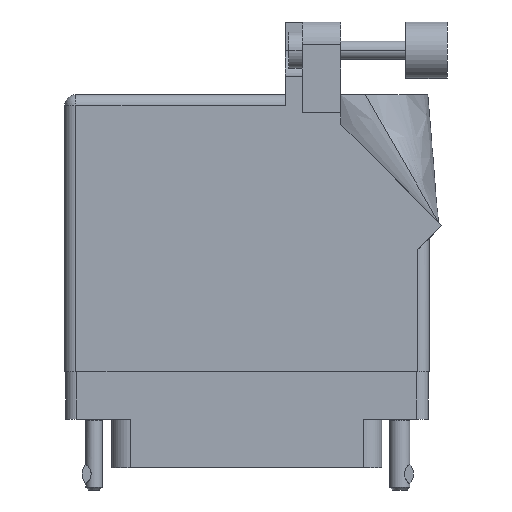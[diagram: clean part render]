
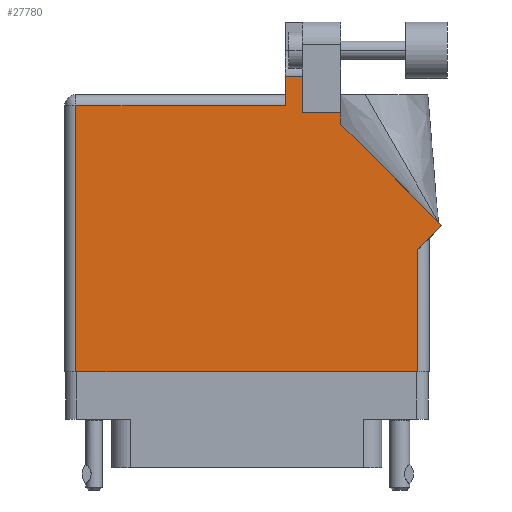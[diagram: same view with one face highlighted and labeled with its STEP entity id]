
A CAD part, front view. The second image highlights one B-rep face of the part: STEP entity #27780.
In plain terms, the highlighted face is planar.
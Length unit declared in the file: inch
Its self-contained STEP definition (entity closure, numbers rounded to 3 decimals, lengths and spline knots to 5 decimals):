
#289 = VECTOR ( 'NONE', #42647, 39.37008 ) ;
#941 = DIRECTION ( 'NONE',  ( 0.707, 0.707, 0. ) ) ;
#992 = DIRECTION ( 'NONE',  ( -0.707, 0.707, 0. ) ) ;
#1466 = VERTEX_POINT ( 'NONE', #11224 ) ;
#1578 = VERTEX_POINT ( 'NONE', #34021 ) ;
#2413 = CARTESIAN_POINT ( 'NONE',  ( 0.062, 0., 0. ) ) ;
#2607 = CARTESIAN_POINT ( 'NONE',  ( 0., 1.53, 0. ) ) ;
#2771 = CARTESIAN_POINT ( 'NONE',  ( 1.64177, 1.6315, 0. ) ) ;
#3176 = LINE ( 'NONE', #9819, #13728 ) ;
#3373 = CARTESIAN_POINT ( 'NONE',  ( 0.062, 0., 0. ) ) ;
#3840 = VECTOR ( 'NONE', #33177, 39.37008 ) ;
#4231 = CARTESIAN_POINT ( 'NONE',  ( 2.01, 0.737, 0. ) ) ;
#5303 = ORIENTED_EDGE ( 'NONE', *, *, #8997, .T. ) ;
#5858 = ORIENTED_EDGE ( 'NONE', *, *, #14724, .T. ) ;
#6082 = EDGE_CURVE ( 'NONE', #47226, #1578, #3176, .T. ) ;
#6361 = LINE ( 'NONE', #26943, #45151 ) ;
#6566 = VERTEX_POINT ( 'NONE', #8274 ) ;
#6800 = CARTESIAN_POINT ( 'NONE',  ( 1.948, 0., 0. ) ) ;
#7767 = VECTOR ( 'NONE', #44574, 39.37008 ) ;
#7984 = LINE ( 'NONE', #3373, #37357 ) ;
#8274 = CARTESIAN_POINT ( 'NONE',  ( 1.217, 1.6315, 0. ) ) ;
#8997 = EDGE_CURVE ( 'NONE', #36861, #6566, #24443, .T. ) ;
#9522 = CARTESIAN_POINT ( 'NONE',  ( 1.948, 0.737, 0. ) ) ;
#9819 = CARTESIAN_POINT ( 'NONE',  ( 1.524, 1.43, 0. ) ) ;
#11224 = CARTESIAN_POINT ( 'NONE',  ( 2.08071, 0.80771, 0. ) ) ;
#11694 = LINE ( 'NONE', #4231, #39904 ) ;
#11801 = CARTESIAN_POINT ( 'NONE',  ( 0.062, 1.468, 0. ) ) ;
#11880 = AXIS2_PLACEMENT_3D ( 'NONE', #2607, #36283, #40048 ) ;
#12091 = ORIENTED_EDGE ( 'NONE', *, *, #28005, .T. ) ;
#12323 = LINE ( 'NONE', #9522, #28180 ) ;
#13728 = VECTOR ( 'NONE', #17634, 39.37008 ) ;
#14170 = VECTOR ( 'NONE', #42451, 39.37008 ) ;
#14499 = CARTESIAN_POINT ( 'NONE',  ( 1.217, 1.468, 0. ) ) ;
#14584 = VECTOR ( 'NONE', #992, 39.37008 ) ;
#14724 = EDGE_CURVE ( 'NONE', #21528, #36771, #12323, .T. ) ;
#16318 = EDGE_CURVE ( 'NONE', #6566, #29069, #6361, .T. ) ;
#17285 = ORIENTED_EDGE ( 'NONE', *, *, #37833, .T. ) ;
#17634 = DIRECTION ( 'NONE',  ( -1., 0., 0. ) ) ;
#17967 = DIRECTION ( 'NONE',  ( 0., -1., 0. ) ) ;
#19061 = EDGE_CURVE ( 'NONE', #47402, #23851, #7984, .T. ) ;
#19409 = EDGE_CURVE ( 'NONE', #43806, #47226, #36724, .T. ) ;
#21252 = LINE ( 'NONE', #36709, #7767 ) ;
#21528 = VERTEX_POINT ( 'NONE', #6800 ) ;
#21964 = CARTESIAN_POINT ( 'NONE',  ( 1.524, 1.43, 0. ) ) ;
#22410 = EDGE_CURVE ( 'NONE', #23851, #21528, #24126, .T. ) ;
#23104 = DIRECTION ( 'NONE',  ( 0., -1., 0. ) ) ;
#23851 = VERTEX_POINT ( 'NONE', #2413 ) ;
#24126 = LINE ( 'NONE', #31111, #14170 ) ;
#24443 = LINE ( 'NONE', #2771, #34416 ) ;
#24554 = LINE ( 'NONE', #41409, #14584 ) ;
#24637 = EDGE_CURVE ( 'NONE', #29069, #47402, #41446, .T. ) ;
#25114 = PLANE ( 'NONE',  #11880 ) ;
#26943 = CARTESIAN_POINT ( 'NONE',  ( 1.217, 1.53, 0. ) ) ;
#27780 = ADVANCED_FACE ( 'NONE', ( #30115 ), #25114, .F. ) ;
#28005 = EDGE_CURVE ( 'NONE', #1578, #36861, #21252, .T. ) ;
#28180 = VECTOR ( 'NONE', #35762, 39.37008 ) ;
#29069 = VERTEX_POINT ( 'NONE', #14499 ) ;
#30115 = FACE_OUTER_BOUND ( 'NONE', #38236, .T. ) ;
#31111 = CARTESIAN_POINT ( 'NONE',  ( 0., 0., 0. ) ) ;
#32686 = ORIENTED_EDGE ( 'NONE', *, *, #43515, .T. ) ;
#33177 = DIRECTION ( 'NONE',  ( -1., 0., 0. ) ) ;
#34021 = CARTESIAN_POINT ( 'NONE',  ( 1.311, 1.43, 0. ) ) ;
#34416 = VECTOR ( 'NONE', #44165, 39.37008 ) ;
#35462 = CARTESIAN_POINT ( 'NONE',  ( 1.524, 1.36442, 0. ) ) ;
#35698 = ORIENTED_EDGE ( 'NONE', *, *, #16318, .T. ) ;
#35762 = DIRECTION ( 'NONE',  ( 0., 1., 0. ) ) ;
#36283 = DIRECTION ( 'NONE',  ( 0., 0., -1. ) ) ;
#36709 = CARTESIAN_POINT ( 'NONE',  ( 1.311, 1.43, 0. ) ) ;
#36724 = LINE ( 'NONE', #46054, #289 ) ;
#36771 = VERTEX_POINT ( 'NONE', #48008 ) ;
#36804 = ORIENTED_EDGE ( 'NONE', *, *, #22410, .T. ) ;
#36861 = VERTEX_POINT ( 'NONE', #45037 ) ;
#37200 = ORIENTED_EDGE ( 'NONE', *, *, #19409, .T. ) ;
#37357 = VECTOR ( 'NONE', #17967, 39.37008 ) ;
#37833 = EDGE_CURVE ( 'NONE', #36771, #1466, #11694, .T. ) ;
#37852 = ORIENTED_EDGE ( 'NONE', *, *, #24637, .T. ) ;
#38236 = EDGE_LOOP ( 'NONE', ( #12091, #5303, #35698, #37852, #47003, #36804, #5858, #17285, #32686, #37200, #46351 ) ) ;
#39904 = VECTOR ( 'NONE', #941, 39.37008 ) ;
#40048 = DIRECTION ( 'NONE',  ( -1., 0., 0. ) ) ;
#40577 = CARTESIAN_POINT ( 'NONE',  ( 0., 1.468, 0. ) ) ;
#41409 = CARTESIAN_POINT ( 'NONE',  ( 2.08071, 0.80771, 0. ) ) ;
#41446 = LINE ( 'NONE', #40577, #3840 ) ;
#42451 = DIRECTION ( 'NONE',  ( 1., 0., 0. ) ) ;
#42647 = DIRECTION ( 'NONE',  ( 0., 1., 0. ) ) ;
#43515 = EDGE_CURVE ( 'NONE', #1466, #43806, #24554, .T. ) ;
#43806 = VERTEX_POINT ( 'NONE', #35462 ) ;
#44165 = DIRECTION ( 'NONE',  ( -1., 0., 0. ) ) ;
#44574 = DIRECTION ( 'NONE',  ( 0., 1., 0. ) ) ;
#45037 = CARTESIAN_POINT ( 'NONE',  ( 1.311, 1.6315, 0. ) ) ;
#45151 = VECTOR ( 'NONE', #23104, 39.37008 ) ;
#46054 = CARTESIAN_POINT ( 'NONE',  ( 1.524, 1.36442, 0. ) ) ;
#46351 = ORIENTED_EDGE ( 'NONE', *, *, #6082, .T. ) ;
#47003 = ORIENTED_EDGE ( 'NONE', *, *, #19061, .T. ) ;
#47226 = VERTEX_POINT ( 'NONE', #21964 ) ;
#47402 = VERTEX_POINT ( 'NONE', #11801 ) ;
#48008 = CARTESIAN_POINT ( 'NONE',  ( 1.948, 0.675, 0. ) ) ;
